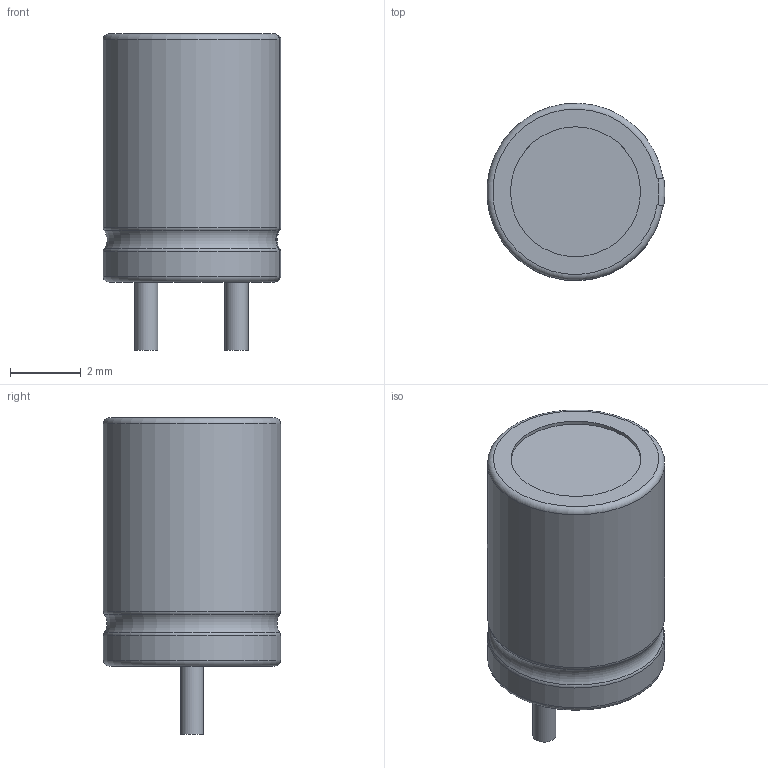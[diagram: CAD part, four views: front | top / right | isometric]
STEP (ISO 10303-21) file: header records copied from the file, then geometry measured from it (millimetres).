
FILE_DESCRIPTION(/* description */ (''),/* implementation_level */ '2;1');
FILE_NAME(/* name */ 'radial_ecap_1583530893362.stp',/* time_stamp */ '2020-03-06T21:41:36+00:00',/* author */ (''),/* organization */ (''),/* preprocessor_version */ 'ST-DEVELOPER v18',/* originating_system */ 'ASM',/* authorisation */ '');
FILE_SCHEMA (('AUTOMOTIVE_DESIGN { 1 0 10303 214 3 1 1 }'));
Length unit declared in the file: millimetre
Products named in the file (1): radial_ecap_1583530893362
Bounding box: 5.01 x 4.99 x 8.92 mm (x, y, z)
Volume: 137 mm3; surface area: 156.6 mm2
Topology: 1 solids, 1 shells, 34 faces, 85 edges, 58 vertices
Faces by surface type: plane 15, torus 10, cylinder 9
Full cylindrical faces by diameter (mm): 0.65 x2, 3.667 x1
Entity records: 1130 total; most frequent: DIRECTION 209, CARTESIAN_POINT 178, ORIENTED_EDGE 170, AXIS2_PLACEMENT_3D 89, EDGE_CURVE 85, VERTEX_POINT 58, CIRCLE 54, EDGE_LOOP 39
